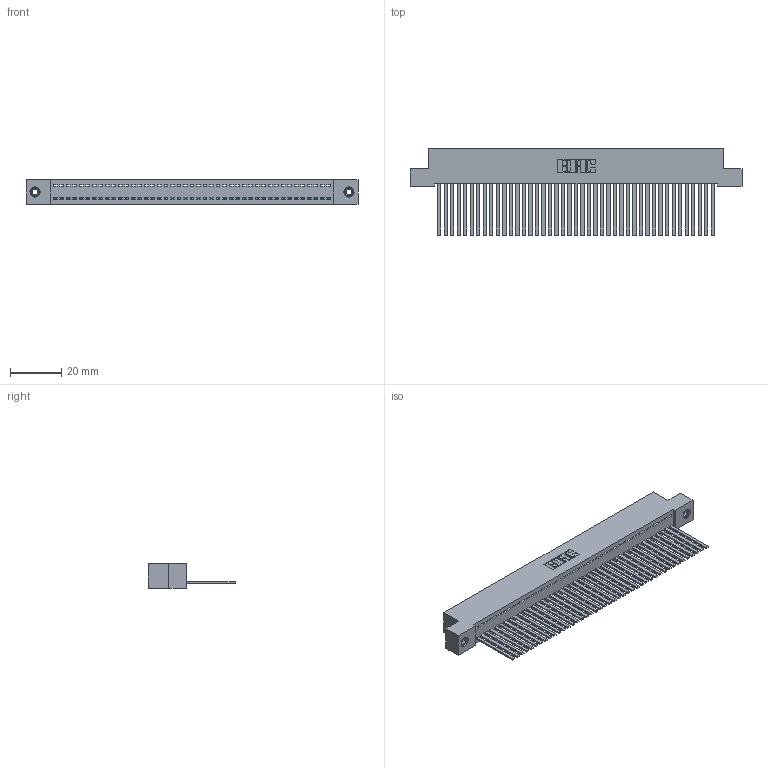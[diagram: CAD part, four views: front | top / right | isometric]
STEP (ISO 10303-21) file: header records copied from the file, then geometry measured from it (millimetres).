
FILE_DESCRIPTION (( 'STEP AP203' ), '1' );
FILE_NAME ('392-043-544-108.STEP', '2019-10-07T21:52:18', ( '' ), ( '' ), 'SwSTEP 2.0', 'SolidWorks 2016', '' );
FILE_SCHEMA (( 'CONFIG_CONTROL_DESIGN' ));
Length unit declared in the file: inch
Products named in the file (4): 392-043-544-108; 342 Part_TI; 345-292-001_345-293-144; 345-250-001_345-250-003-102
Assembly tree (46 placements, depth 2):
  392-043-544-108
    342 Part_TI
    345-292-001_345-293-144  x43
    345-250-001_345-250-003-102  x2
Bounding box: 129.54 x 34.3 x 9.4 mm (x, y, z)
Volume: 11854.1 mm3; surface area: 18861 mm2
Topology: 46 solids, 46 shells, 2406 faces, 7229 edges, 4754 vertices
Faces by surface type: plane 1732, cylinder 658, cone 12, torus 4
Entity records: 27028 total; most frequent: CARTESIAN_POINT 4642, ORIENTED_EDGE 4614, DIRECTION 3943, EDGE_CURVE 2307, LINE 2163, VECTOR 2163, VERTEX_POINT 1532, AXIS2_PLACEMENT_3D 890
